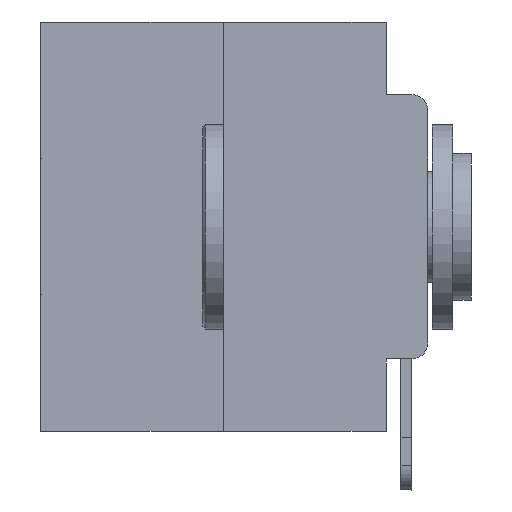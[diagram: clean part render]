
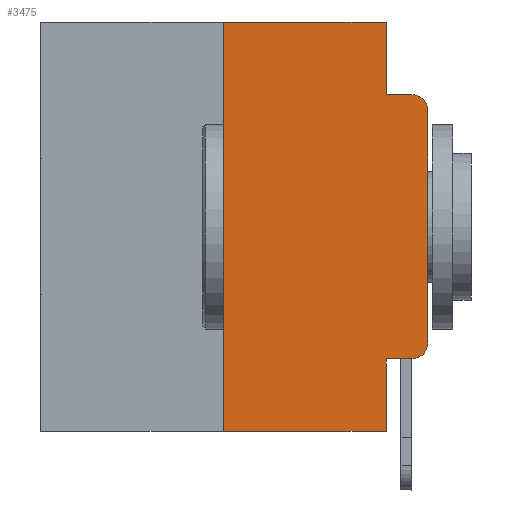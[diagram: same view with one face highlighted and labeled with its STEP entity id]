
A CAD part, left-side view. The second image highlights one B-rep face of the part: STEP entity #3475.
In plain terms, the highlighted planar face has unit normal (-1, 0, 0).
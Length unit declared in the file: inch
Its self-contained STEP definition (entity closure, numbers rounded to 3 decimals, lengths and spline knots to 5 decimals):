
#124 = CARTESIAN_POINT ( 'NONE',  ( 0., 0.25, 0. ) ) ;
#259 = EDGE_CURVE ( 'NONE', #24426, #22199, #9114, .T. ) ;
#262 = VERTEX_POINT ( 'NONE', #6329 ) ;
#852 = CARTESIAN_POINT ( 'NONE',  ( 0., 0.473, -0.5 ) ) ;
#1025 = ORIENTED_EDGE ( 'NONE', *, *, #20830, .F. ) ;
#1092 = VERTEX_POINT ( 'NONE', #5543 ) ;
#1574 = CARTESIAN_POINT ( 'NONE',  ( 0., 0.02, -0.3915 ) ) ;
#1856 = DIRECTION ( 'NONE',  ( 0., 0., -1. ) ) ;
#2134 = CARTESIAN_POINT ( 'NONE',  ( 0., 0., 0. ) ) ;
#2339 = VECTOR ( 'NONE', #16910, 39.37008 ) ;
#3475 = ADVANCED_FACE ( 'NONE', ( #27178 ), #27028, .F. ) ;
#3571 = EDGE_CURVE ( 'NONE', #8087, #1092, #21271, .T. ) ;
#4074 = CARTESIAN_POINT ( 'NONE',  ( 0., 0.051, -0.0885 ) ) ;
#4582 = DIRECTION ( 'NONE',  ( 0., -1., 0. ) ) ;
#4693 = VERTEX_POINT ( 'NONE', #124 ) ;
#5543 = CARTESIAN_POINT ( 'NONE',  ( 0., 0.051, -0.5 ) ) ;
#6326 = CARTESIAN_POINT ( 'NONE',  ( 0., 0.473, 0. ) ) ;
#6329 = CARTESIAN_POINT ( 'NONE',  ( 0., 0.051, -0.4115 ) ) ;
#6759 = DIRECTION ( 'NONE',  ( 0., 0., -1. ) ) ;
#7411 = ORIENTED_EDGE ( 'NONE', *, *, #3571, .T. ) ;
#7620 = VECTOR ( 'NONE', #8485, 39.37008 ) ;
#7656 = EDGE_CURVE ( 'NONE', #262, #13140, #9253, .T. ) ;
#7951 = EDGE_CURVE ( 'NONE', #17325, #24426, #11011, .T. ) ;
#8087 = VERTEX_POINT ( 'NONE', #25888 ) ;
#8351 = VECTOR ( 'NONE', #8771, 39.37008 ) ;
#8485 = DIRECTION ( 'NONE',  ( 0., -1., 0. ) ) ;
#8771 = DIRECTION ( 'NONE',  ( 0., 0., 1. ) ) ;
#9023 = EDGE_CURVE ( 'NONE', #4693, #20895, #11172, .T. ) ;
#9114 = CIRCLE ( 'NONE', #22350, 0.02 ) ;
#9253 = LINE ( 'NONE', #26242, #17008 ) ;
#9348 = EDGE_CURVE ( 'NONE', #20895, #11009, #18852, .T. ) ;
#9518 = ORIENTED_EDGE ( 'NONE', *, *, #13443, .T. ) ;
#9962 = DIRECTION ( 'NONE',  ( 0., 0., -1. ) ) ;
#10132 = DIRECTION ( 'NONE',  ( 0., -1., 0. ) ) ;
#11009 = VERTEX_POINT ( 'NONE', #4074 ) ;
#11011 = LINE ( 'NONE', #2134, #8351 ) ;
#11168 = ORIENTED_EDGE ( 'NONE', *, *, #9348, .F. ) ;
#11172 = LINE ( 'NONE', #12965, #7620 ) ;
#11570 = AXIS2_PLACEMENT_3D ( 'NONE', #1574, #22127, #1856 ) ;
#12041 = LINE ( 'NONE', #21056, #2339 ) ;
#12047 = CIRCLE ( 'NONE', #11570, 0.02 ) ;
#12624 = DIRECTION ( 'NONE',  ( 0., 0., -1. ) ) ;
#12965 = CARTESIAN_POINT ( 'NONE',  ( 0., 0.473, 0. ) ) ;
#13140 = VERTEX_POINT ( 'NONE', #27171 ) ;
#13443 = EDGE_CURVE ( 'NONE', #13140, #17325, #12047, .T. ) ;
#15004 = VECTOR ( 'NONE', #12624, 39.37008 ) ;
#16015 = ORIENTED_EDGE ( 'NONE', *, *, #259, .T. ) ;
#16693 = DIRECTION ( 'NONE',  ( 0., -1., 0. ) ) ;
#16781 = CARTESIAN_POINT ( 'NONE',  ( 0., 0.051, 0. ) ) ;
#16910 = DIRECTION ( 'NONE',  ( 0., 0., 1. ) ) ;
#17008 = VECTOR ( 'NONE', #10132, 39.37008 ) ;
#17325 = VERTEX_POINT ( 'NONE', #24263 ) ;
#17981 = VECTOR ( 'NONE', #16693, 39.37008 ) ;
#18039 = CARTESIAN_POINT ( 'NONE',  ( 0., 0.02, -0.1085 ) ) ;
#18852 = LINE ( 'NONE', #16781, #28909 ) ;
#19087 = CARTESIAN_POINT ( 'NONE',  ( 0., 0.051, 0. ) ) ;
#19428 = LINE ( 'NONE', #26064, #15004 ) ;
#19436 = ORIENTED_EDGE ( 'NONE', *, *, #7656, .T. ) ;
#20276 = LINE ( 'NONE', #20420, #27571 ) ;
#20420 = CARTESIAN_POINT ( 'NONE',  ( 0., 0.051, -0.0885 ) ) ;
#20432 = CARTESIAN_POINT ( 'NONE',  ( 0., 0., -0.1085 ) ) ;
#20830 = EDGE_CURVE ( 'NONE', #11009, #22199, #20276, .T. ) ;
#20895 = VERTEX_POINT ( 'NONE', #19087 ) ;
#21022 = ORIENTED_EDGE ( 'NONE', *, *, #27980, .F. ) ;
#21056 = CARTESIAN_POINT ( 'NONE',  ( 0., 0.25, 0. ) ) ;
#21271 = LINE ( 'NONE', #852, #17981 ) ;
#22029 = DIRECTION ( 'NONE',  ( -1., 0., 0. ) ) ;
#22127 = DIRECTION ( 'NONE',  ( -1., 0., 0. ) ) ;
#22175 = DIRECTION ( 'NONE',  ( 1., 0., 0. ) ) ;
#22199 = VERTEX_POINT ( 'NONE', #25045 ) ;
#22350 = AXIS2_PLACEMENT_3D ( 'NONE', #18039, #22029, #27031 ) ;
#24263 = CARTESIAN_POINT ( 'NONE',  ( 0., 0., -0.3915 ) ) ;
#24426 = VERTEX_POINT ( 'NONE', #20432 ) ;
#24739 = EDGE_LOOP ( 'NONE', ( #25496, #16015, #1025, #11168, #25027, #21022, #7411, #27219, #19436, #9518 ) ) ;
#25027 = ORIENTED_EDGE ( 'NONE', *, *, #9023, .F. ) ;
#25045 = CARTESIAN_POINT ( 'NONE',  ( 0., 0.02, -0.0885 ) ) ;
#25444 = EDGE_CURVE ( 'NONE', #262, #1092, #19428, .T. ) ;
#25496 = ORIENTED_EDGE ( 'NONE', *, *, #7951, .T. ) ;
#25888 = CARTESIAN_POINT ( 'NONE',  ( 0., 0.25, -0.5 ) ) ;
#25968 = AXIS2_PLACEMENT_3D ( 'NONE', #6326, #22175, #6759 ) ;
#26064 = CARTESIAN_POINT ( 'NONE',  ( 0., 0.051, 0. ) ) ;
#26242 = CARTESIAN_POINT ( 'NONE',  ( 0., 0.051, -0.4115 ) ) ;
#27028 = PLANE ( 'NONE',  #25968 ) ;
#27031 = DIRECTION ( 'NONE',  ( 0., 0., -1. ) ) ;
#27171 = CARTESIAN_POINT ( 'NONE',  ( 0., 0.02, -0.4115 ) ) ;
#27178 = FACE_OUTER_BOUND ( 'NONE', #24739, .T. ) ;
#27219 = ORIENTED_EDGE ( 'NONE', *, *, #25444, .F. ) ;
#27571 = VECTOR ( 'NONE', #4582, 39.37008 ) ;
#27980 = EDGE_CURVE ( 'NONE', #8087, #4693, #12041, .T. ) ;
#28909 = VECTOR ( 'NONE', #9962, 39.37008 ) ;
